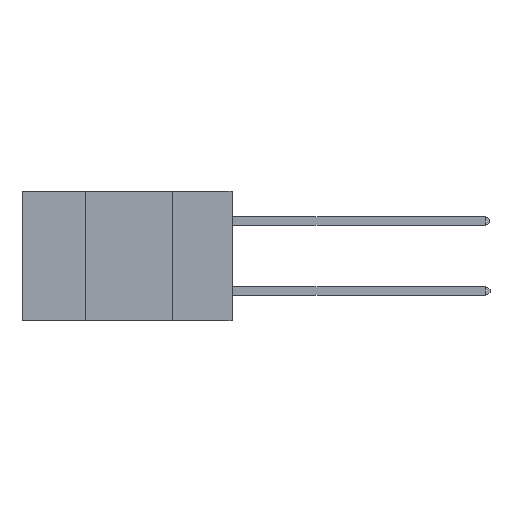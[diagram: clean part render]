
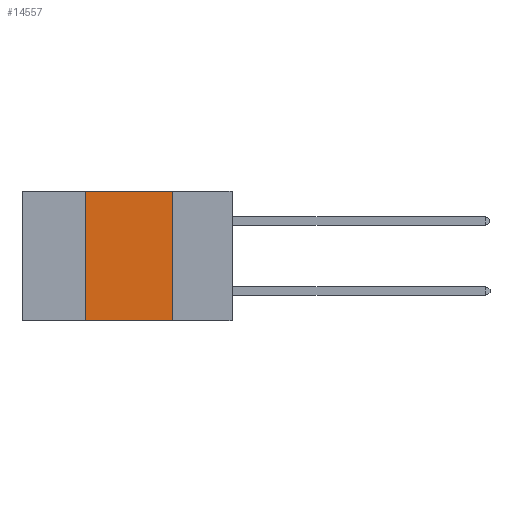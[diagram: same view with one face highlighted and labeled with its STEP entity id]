
A CAD part, left-side view. The second image highlights one B-rep face of the part: STEP entity #14557.
In plain terms, the highlighted planar face has unit normal (-1, 0, 0).
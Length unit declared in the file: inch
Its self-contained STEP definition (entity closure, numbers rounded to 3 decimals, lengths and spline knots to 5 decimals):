
#6 = LINE ( 'NONE', #16042, #3243 ) ;
#166 = PLANE ( 'NONE',  #4471 ) ;
#330 = VERTEX_POINT ( 'NONE', #6730 ) ;
#1112 = VERTEX_POINT ( 'NONE', #10463 ) ;
#2793 = CARTESIAN_POINT ( 'NONE',  ( 0., 0.42, 0. ) ) ;
#2911 = DIRECTION ( 'NONE',  ( 0., 0., -1. ) ) ;
#3243 = VECTOR ( 'NONE', #12262, 39.37008 ) ;
#3438 = VECTOR ( 'NONE', #16401, 39.37008 ) ;
#4471 = AXIS2_PLACEMENT_3D ( 'NONE', #15802, #10755, #2911 ) ;
#4499 = ORIENTED_EDGE ( 'NONE', *, *, #16198, .T. ) ;
#4564 = EDGE_LOOP ( 'NONE', ( #14665, #13391, #16639, #4499 ) ) ;
#6145 = EDGE_CURVE ( 'NONE', #11279, #330, #7419, .T. ) ;
#6730 = CARTESIAN_POINT ( 'NONE',  ( 0., 0.17, 0. ) ) ;
#6901 = LINE ( 'NONE', #2793, #7731 ) ;
#7072 = LINE ( 'NONE', #10107, #3438 ) ;
#7323 = CARTESIAN_POINT ( 'NONE',  ( 0., 0.6, 0. ) ) ;
#7419 = LINE ( 'NONE', #7323, #13613 ) ;
#7731 = VECTOR ( 'NONE', #11910, 39.37008 ) ;
#8465 = CARTESIAN_POINT ( 'NONE',  ( 0., 0.17, -0.37 ) ) ;
#8599 = DIRECTION ( 'NONE',  ( 0., -1., 0. ) ) ;
#10107 = CARTESIAN_POINT ( 'NONE',  ( 0., 0.6, -0.37 ) ) ;
#10463 = CARTESIAN_POINT ( 'NONE',  ( 0., 0.42, -0.37 ) ) ;
#10755 = DIRECTION ( 'NONE',  ( 1., 0., 0. ) ) ;
#11279 = VERTEX_POINT ( 'NONE', #14426 ) ;
#11910 = DIRECTION ( 'NONE',  ( 0., 0., 1. ) ) ;
#12262 = DIRECTION ( 'NONE',  ( 0., 0., -1. ) ) ;
#12754 = FACE_OUTER_BOUND ( 'NONE', #4564, .T. ) ;
#13391 = ORIENTED_EDGE ( 'NONE', *, *, #6145, .F. ) ;
#13613 = VECTOR ( 'NONE', #8599, 39.37008 ) ;
#14192 = VERTEX_POINT ( 'NONE', #8465 ) ;
#14426 = CARTESIAN_POINT ( 'NONE',  ( 0., 0.42, 0. ) ) ;
#14498 = EDGE_CURVE ( 'NONE', #1112, #11279, #6901, .T. ) ;
#14557 = ADVANCED_FACE ( 'NONE', ( #12754 ), #166, .F. ) ;
#14665 = ORIENTED_EDGE ( 'NONE', *, *, #15348, .F. ) ;
#15348 = EDGE_CURVE ( 'NONE', #330, #14192, #6, .T. ) ;
#15802 = CARTESIAN_POINT ( 'NONE',  ( 0., 0.6, 0. ) ) ;
#16042 = CARTESIAN_POINT ( 'NONE',  ( 0., 0.17, 0. ) ) ;
#16198 = EDGE_CURVE ( 'NONE', #1112, #14192, #7072, .T. ) ;
#16401 = DIRECTION ( 'NONE',  ( 0., -1., 0. ) ) ;
#16639 = ORIENTED_EDGE ( 'NONE', *, *, #14498, .F. ) ;
